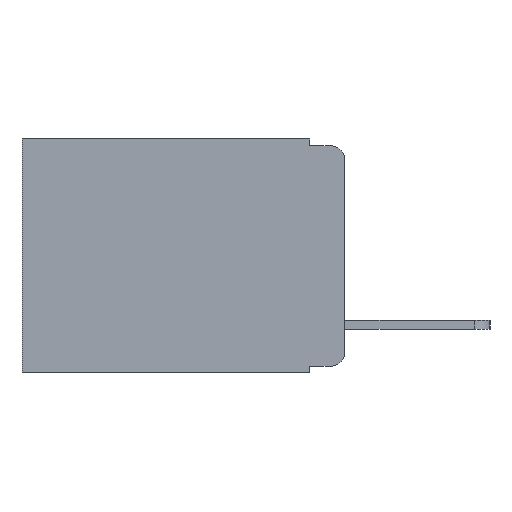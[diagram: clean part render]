
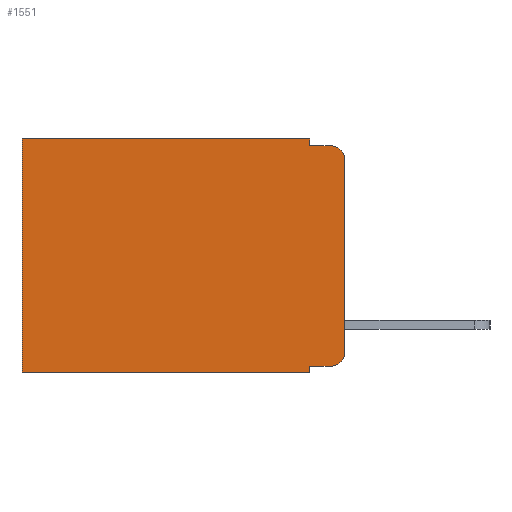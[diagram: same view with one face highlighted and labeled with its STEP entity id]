
A CAD part, left-side view. The second image highlights one B-rep face of the part: STEP entity #1551.
In plain terms, the highlighted planar face has unit normal (-1, 0, 0).
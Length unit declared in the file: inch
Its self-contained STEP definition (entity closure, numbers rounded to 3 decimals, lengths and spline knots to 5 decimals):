
#228 = AXIS2_PLACEMENT_3D ( 'NONE', #2983, #2966, #1355 ) ;
#237 = CARTESIAN_POINT ( 'NONE',  ( 0.298, 0.473, 0. ) ) ;
#327 = CARTESIAN_POINT ( 'NONE',  ( 0.298, 0., 0. ) ) ;
#354 = DIRECTION ( 'NONE',  ( 0., 0., -1. ) ) ;
#477 = VERTEX_POINT ( 'NONE', #3300 ) ;
#501 = VECTOR ( 'NONE', #7700, 39.37008 ) ;
#744 = LINE ( 'NONE', #5176, #501 ) ;
#926 = VERTEX_POINT ( 'NONE', #5993 ) ;
#945 = VECTOR ( 'NONE', #6324, 39.37008 ) ;
#1047 = LINE ( 'NONE', #6269, #945 ) ;
#1169 = VERTEX_POINT ( 'NONE', #3456 ) ;
#1234 = VERTEX_POINT ( 'NONE', #7326 ) ;
#1355 = DIRECTION ( 'NONE',  ( 0., 0., -1. ) ) ;
#1377 = EDGE_LOOP ( 'NONE', ( #2434, #2571, #2731, #2911, #2940, #3063, #3075, #3216, #3414, #3504 ) ) ;
#1551 = ADVANCED_FACE ( 'NONE', ( #6726 ), #7486, .F. ) ;
#1736 = VERTEX_POINT ( 'NONE', #5362 ) ;
#1979 = VERTEX_POINT ( 'NONE', #10546 ) ;
#2092 = DIRECTION ( 'NONE',  ( 0., -1., 0. ) ) ;
#2434 = ORIENTED_EDGE ( 'NONE', *, *, #2669, .F. ) ;
#2571 = ORIENTED_EDGE ( 'NONE', *, *, #2774, .T. ) ;
#2669 = EDGE_CURVE ( 'NONE', #11957, #1979, #8852, .T. ) ;
#2731 = ORIENTED_EDGE ( 'NONE', *, *, #3453, .F. ) ;
#2774 = EDGE_CURVE ( 'NONE', #11957, #3488, #8156, .T. ) ;
#2910 = DIRECTION ( 'NONE',  ( 0., 0., -1. ) ) ;
#2911 = ORIENTED_EDGE ( 'NONE', *, *, #4366, .F. ) ;
#2940 = ORIENTED_EDGE ( 'NONE', *, *, #10374, .T. ) ;
#2966 = DIRECTION ( 'NONE',  ( -1., 0., 0. ) ) ;
#2983 = CARTESIAN_POINT ( 'NONE',  ( 0.298, 0.02, -0.313 ) ) ;
#2994 = LINE ( 'NONE', #237, #7638 ) ;
#3063 = ORIENTED_EDGE ( 'NONE', *, *, #4757, .T. ) ;
#3064 = CARTESIAN_POINT ( 'NONE',  ( 0.298, 0., -0.03 ) ) ;
#3075 = ORIENTED_EDGE ( 'NONE', *, *, #4322, .F. ) ;
#3216 = ORIENTED_EDGE ( 'NONE', *, *, #4784, .F. ) ;
#3300 = CARTESIAN_POINT ( 'NONE',  ( 0.298, 0.051, -0.333 ) ) ;
#3414 = ORIENTED_EDGE ( 'NONE', *, *, #4800, .T. ) ;
#3453 = EDGE_CURVE ( 'NONE', #1169, #3488, #4587, .T. ) ;
#3456 = CARTESIAN_POINT ( 'NONE',  ( 0.298, 0.051, -0.01 ) ) ;
#3488 = VERTEX_POINT ( 'NONE', #9880 ) ;
#3500 = CARTESIAN_POINT ( 'NONE',  ( 0.298, 0.051, -0.333 ) ) ;
#3503 = CIRCLE ( 'NONE', #228, 0.02 ) ;
#3504 = ORIENTED_EDGE ( 'NONE', *, *, #4990, .T. ) ;
#3678 = AXIS2_PLACEMENT_3D ( 'NONE', #9668, #9900, #354 ) ;
#3744 = DIRECTION ( 'NONE',  ( 0., -1., 0. ) ) ;
#3784 = DIRECTION ( 'NONE',  ( 0., 0., -1. ) ) ;
#4025 = DIRECTION ( 'NONE',  ( 0., 0., -1. ) ) ;
#4322 = EDGE_CURVE ( 'NONE', #1234, #926, #1047, .T. ) ;
#4366 = EDGE_CURVE ( 'NONE', #5348, #1169, #744, .T. ) ;
#4460 = LINE ( 'NONE', #11780, #11034 ) ;
#4481 = VECTOR ( 'NONE', #3744, 39.37008 ) ;
#4587 = LINE ( 'NONE', #5870, #4481 ) ;
#4757 = EDGE_CURVE ( 'NONE', #5624, #926, #2994, .T. ) ;
#4784 = EDGE_CURVE ( 'NONE', #477, #1234, #5549, .T. ) ;
#4800 = EDGE_CURVE ( 'NONE', #477, #1736, #7376, .T. ) ;
#4990 = EDGE_CURVE ( 'NONE', #1736, #1979, #3503, .T. ) ;
#5176 = CARTESIAN_POINT ( 'NONE',  ( 0.298, 0.051, 0. ) ) ;
#5348 = VERTEX_POINT ( 'NONE', #11658 ) ;
#5362 = CARTESIAN_POINT ( 'NONE',  ( 0.298, 0.02, -0.333 ) ) ;
#5549 = LINE ( 'NONE', #7323, #9638 ) ;
#5624 = VERTEX_POINT ( 'NONE', #10034 ) ;
#5870 = CARTESIAN_POINT ( 'NONE',  ( 0.298, 0.051, -0.01 ) ) ;
#5993 = CARTESIAN_POINT ( 'NONE',  ( 0.298, 0.473, -0.343 ) ) ;
#6269 = CARTESIAN_POINT ( 'NONE',  ( 0.298, 0., -0.343 ) ) ;
#6324 = DIRECTION ( 'NONE',  ( 0., 1., 0. ) ) ;
#6726 = FACE_OUTER_BOUND ( 'NONE', #1377, .T. ) ;
#7323 = CARTESIAN_POINT ( 'NONE',  ( 0.298, 0.051, 0. ) ) ;
#7326 = CARTESIAN_POINT ( 'NONE',  ( 0.298, 0.051, -0.343 ) ) ;
#7376 = LINE ( 'NONE', #3500, #11489 ) ;
#7451 = DIRECTION ( 'NONE',  ( 0., 0., -1. ) ) ;
#7462 = DIRECTION ( 'NONE',  ( 1., 0., 0. ) ) ;
#7486 = PLANE ( 'NONE',  #10527 ) ;
#7638 = VECTOR ( 'NONE', #4025, 39.37008 ) ;
#7700 = DIRECTION ( 'NONE',  ( 0., 0., -1. ) ) ;
#7825 = CARTESIAN_POINT ( 'NONE',  ( 0.298, 0., 0. ) ) ;
#8156 = CIRCLE ( 'NONE', #3678, 0.02 ) ;
#8809 = VECTOR ( 'NONE', #2910, 39.37008 ) ;
#8852 = LINE ( 'NONE', #327, #8809 ) ;
#9638 = VECTOR ( 'NONE', #3784, 39.37008 ) ;
#9668 = CARTESIAN_POINT ( 'NONE',  ( 0.298, 0.02, -0.03 ) ) ;
#9880 = CARTESIAN_POINT ( 'NONE',  ( 0.298, 0.02, -0.01 ) ) ;
#9900 = DIRECTION ( 'NONE',  ( -1., 0., 0. ) ) ;
#10034 = CARTESIAN_POINT ( 'NONE',  ( 0.298, 0.473, 0. ) ) ;
#10374 = EDGE_CURVE ( 'NONE', #5348, #5624, #4460, .T. ) ;
#10527 = AXIS2_PLACEMENT_3D ( 'NONE', #7825, #7462, #7451 ) ;
#10546 = CARTESIAN_POINT ( 'NONE',  ( 0.298, 0., -0.313 ) ) ;
#11034 = VECTOR ( 'NONE', #11728, 39.37008 ) ;
#11489 = VECTOR ( 'NONE', #2092, 39.37008 ) ;
#11658 = CARTESIAN_POINT ( 'NONE',  ( 0.298, 0.051, 0. ) ) ;
#11728 = DIRECTION ( 'NONE',  ( 0., 1., 0. ) ) ;
#11780 = CARTESIAN_POINT ( 'NONE',  ( 0.298, 0., 0. ) ) ;
#11957 = VERTEX_POINT ( 'NONE', #3064 ) ;
